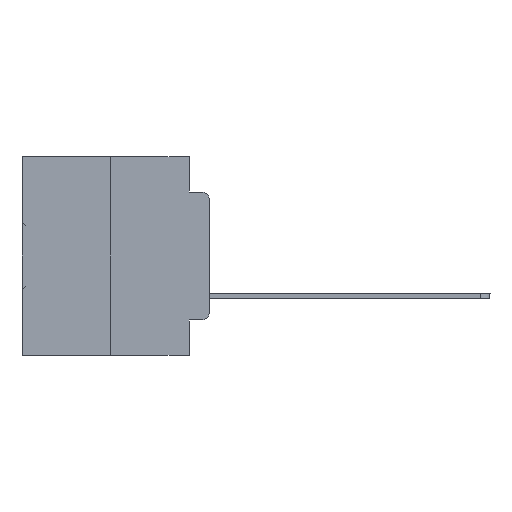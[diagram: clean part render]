
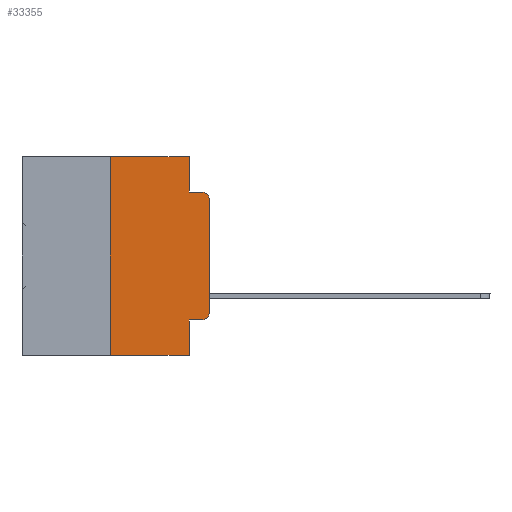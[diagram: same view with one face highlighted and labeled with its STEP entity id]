
A CAD part, left-side view. The second image highlights one B-rep face of the part: STEP entity #33355.
In plain terms, the highlighted planar face has unit normal (-1, 0, 0).
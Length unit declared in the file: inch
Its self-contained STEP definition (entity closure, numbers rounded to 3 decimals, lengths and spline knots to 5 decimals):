
#99 = EDGE_CURVE ( 'NONE', #10622, #8798, #7573, .T. ) ;
#200 = EDGE_CURVE ( 'NONE', #6216, #1509, #24837, .T. ) ;
#266 = DIRECTION ( 'NONE',  ( 0., 0., 1. ) ) ;
#272 = CARTESIAN_POINT ( 'NONE',  ( 0., 0., -0.3915 ) ) ;
#559 = CARTESIAN_POINT ( 'NONE',  ( 0., 0.25, 0. ) ) ;
#561 = DIRECTION ( 'NONE',  ( 0., 0., -1. ) ) ;
#628 = CARTESIAN_POINT ( 'NONE',  ( 0., 0.473, 0. ) ) ;
#1509 = VERTEX_POINT ( 'NONE', #30096 ) ;
#2108 = CARTESIAN_POINT ( 'NONE',  ( 0., 0.02, -0.4115 ) ) ;
#2839 = DIRECTION ( 'NONE',  ( 0., 0., -1. ) ) ;
#3071 = VECTOR ( 'NONE', #33423, 39.37008 ) ;
#3297 = AXIS2_PLACEMENT_3D ( 'NONE', #28805, #4067, #2839 ) ;
#4067 = DIRECTION ( 'NONE',  ( 1., 0., 0. ) ) ;
#5637 = VECTOR ( 'NONE', #33757, 39.37008 ) ;
#6216 = VERTEX_POINT ( 'NONE', #33437 ) ;
#6248 = DIRECTION ( 'NONE',  ( 0., -1., 0. ) ) ;
#6404 = VECTOR ( 'NONE', #11124, 39.37008 ) ;
#6790 = FACE_OUTER_BOUND ( 'NONE', #7243, .T. ) ;
#7243 = EDGE_LOOP ( 'NONE', ( #23674, #32468, #26062, #12741, #34495, #27718, #20796, #32629, #24157, #26655 ) ) ;
#7573 = CIRCLE ( 'NONE', #13360, 0.02 ) ;
#8786 = EDGE_CURVE ( 'NONE', #13813, #20239, #33132, .T. ) ;
#8798 = VERTEX_POINT ( 'NONE', #272 ) ;
#9240 = EDGE_CURVE ( 'NONE', #6216, #10622, #14847, .T. ) ;
#10595 = DIRECTION ( 'NONE',  ( 0., 0., -1. ) ) ;
#10622 = VERTEX_POINT ( 'NONE', #2108 ) ;
#11124 = DIRECTION ( 'NONE',  ( 0., 0., -1. ) ) ;
#11259 = CARTESIAN_POINT ( 'NONE',  ( 0., 0.051, 0. ) ) ;
#11476 = CARTESIAN_POINT ( 'NONE',  ( 0., 0., -0.1085 ) ) ;
#12166 = DIRECTION ( 'NONE',  ( 0., -1., 0. ) ) ;
#12741 = ORIENTED_EDGE ( 'NONE', *, *, #25588, .F. ) ;
#12827 = VERTEX_POINT ( 'NONE', #24231 ) ;
#13360 = AXIS2_PLACEMENT_3D ( 'NONE', #26850, #32433, #15876 ) ;
#13658 = EDGE_CURVE ( 'NONE', #12827, #1509, #32802, .T. ) ;
#13813 = VERTEX_POINT ( 'NONE', #21282 ) ;
#14285 = EDGE_CURVE ( 'NONE', #17461, #23534, #17103, .T. ) ;
#14847 = LINE ( 'NONE', #22759, #5637 ) ;
#15876 = DIRECTION ( 'NONE',  ( 0., 0., -1. ) ) ;
#16244 = DIRECTION ( 'NONE',  ( 0., -1., 0. ) ) ;
#16507 = AXIS2_PLACEMENT_3D ( 'NONE', #25669, #31257, #561 ) ;
#17103 = CIRCLE ( 'NONE', #16507, 0.02 ) ;
#17461 = VERTEX_POINT ( 'NONE', #11476 ) ;
#17819 = PLANE ( 'NONE',  #3297 ) ;
#18522 = VECTOR ( 'NONE', #6248, 39.37008 ) ;
#18615 = EDGE_CURVE ( 'NONE', #8798, #17461, #25552, .T. ) ;
#19043 = EDGE_CURVE ( 'NONE', #26708, #23534, #20655, .T. ) ;
#19562 = LINE ( 'NONE', #559, #3071 ) ;
#20153 = VECTOR ( 'NONE', #10595, 39.37008 ) ;
#20239 = VERTEX_POINT ( 'NONE', #11259 ) ;
#20655 = LINE ( 'NONE', #33800, #31380 ) ;
#20796 = ORIENTED_EDGE ( 'NONE', *, *, #13658, .T. ) ;
#21282 = CARTESIAN_POINT ( 'NONE',  ( 0., 0.25, 0. ) ) ;
#21648 = VECTOR ( 'NONE', #266, 39.37008 ) ;
#21956 = CARTESIAN_POINT ( 'NONE',  ( 0., 0.051, 0. ) ) ;
#21967 = CARTESIAN_POINT ( 'NONE',  ( 0., 0.051, -0.0885 ) ) ;
#22759 = CARTESIAN_POINT ( 'NONE',  ( 0., 0.051, -0.4115 ) ) ;
#23534 = VERTEX_POINT ( 'NONE', #32338 ) ;
#23674 = ORIENTED_EDGE ( 'NONE', *, *, #18615, .T. ) ;
#23777 = CARTESIAN_POINT ( 'NONE',  ( 0., 0.051, 0. ) ) ;
#24157 = ORIENTED_EDGE ( 'NONE', *, *, #9240, .T. ) ;
#24231 = CARTESIAN_POINT ( 'NONE',  ( 0., 0.25, -0.5 ) ) ;
#24802 = VECTOR ( 'NONE', #16244, 39.37008 ) ;
#24837 = LINE ( 'NONE', #21956, #6404 ) ;
#25552 = LINE ( 'NONE', #30785, #21648 ) ;
#25588 = EDGE_CURVE ( 'NONE', #20239, #26708, #35313, .T. ) ;
#25669 = CARTESIAN_POINT ( 'NONE',  ( 0., 0.02, -0.1085 ) ) ;
#26062 = ORIENTED_EDGE ( 'NONE', *, *, #19043, .F. ) ;
#26655 = ORIENTED_EDGE ( 'NONE', *, *, #99, .T. ) ;
#26708 = VERTEX_POINT ( 'NONE', #21967 ) ;
#26850 = CARTESIAN_POINT ( 'NONE',  ( 0., 0.02, -0.3915 ) ) ;
#27718 = ORIENTED_EDGE ( 'NONE', *, *, #27742, .F. ) ;
#27742 = EDGE_CURVE ( 'NONE', #12827, #13813, #19562, .T. ) ;
#28805 = CARTESIAN_POINT ( 'NONE',  ( 0., 0.473, 0. ) ) ;
#30096 = CARTESIAN_POINT ( 'NONE',  ( 0., 0.051, -0.5 ) ) ;
#30785 = CARTESIAN_POINT ( 'NONE',  ( 0., 0., 0. ) ) ;
#31257 = DIRECTION ( 'NONE',  ( -1., 0., 0. ) ) ;
#31380 = VECTOR ( 'NONE', #12166, 39.37008 ) ;
#32338 = CARTESIAN_POINT ( 'NONE',  ( 0., 0.02, -0.0885 ) ) ;
#32433 = DIRECTION ( 'NONE',  ( -1., 0., 0. ) ) ;
#32468 = ORIENTED_EDGE ( 'NONE', *, *, #14285, .T. ) ;
#32629 = ORIENTED_EDGE ( 'NONE', *, *, #200, .F. ) ;
#32802 = LINE ( 'NONE', #35334, #24802 ) ;
#33132 = LINE ( 'NONE', #628, #18522 ) ;
#33355 = ADVANCED_FACE ( 'NONE', ( #6790 ), #17819, .F. ) ;
#33423 = DIRECTION ( 'NONE',  ( 0., 0., 1. ) ) ;
#33437 = CARTESIAN_POINT ( 'NONE',  ( 0., 0.051, -0.4115 ) ) ;
#33757 = DIRECTION ( 'NONE',  ( 0., -1., 0. ) ) ;
#33800 = CARTESIAN_POINT ( 'NONE',  ( 0., 0.051, -0.0885 ) ) ;
#34495 = ORIENTED_EDGE ( 'NONE', *, *, #8786, .F. ) ;
#35313 = LINE ( 'NONE', #23777, #20153 ) ;
#35334 = CARTESIAN_POINT ( 'NONE',  ( 0., 0.473, -0.5 ) ) ;
